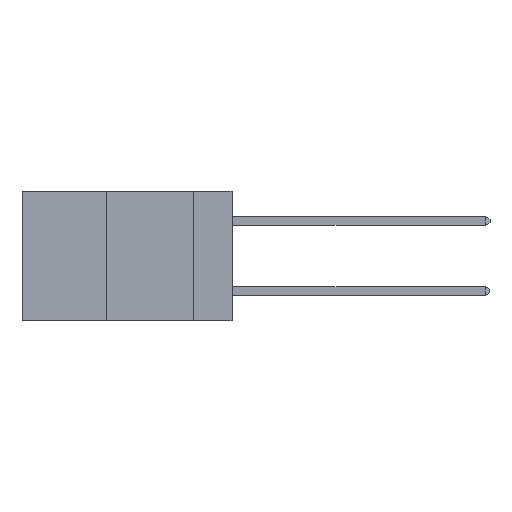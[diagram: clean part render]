
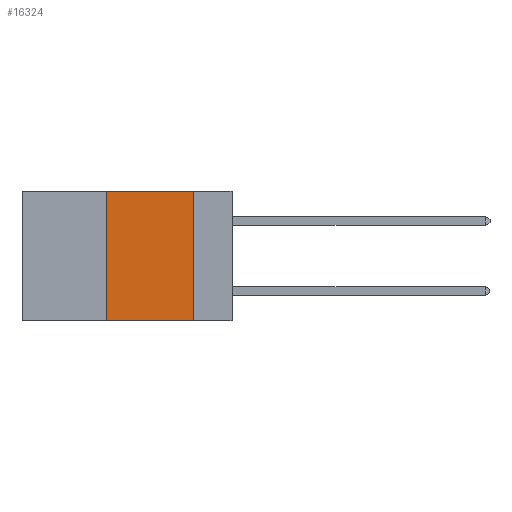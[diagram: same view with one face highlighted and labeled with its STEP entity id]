
A CAD part, left-side view. The second image highlights one B-rep face of the part: STEP entity #16324.
In plain terms, the highlighted planar face has unit normal (-1, 0, 0).
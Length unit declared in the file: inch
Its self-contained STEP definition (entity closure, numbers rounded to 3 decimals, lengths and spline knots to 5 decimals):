
#445 = VECTOR ( 'NONE', #5398, 39.37008 ) ;
#1296 = EDGE_CURVE ( 'NONE', #1911, #14164, #7550, .T. ) ;
#1616 = CARTESIAN_POINT ( 'NONE',  ( 0., 0.6, 0. ) ) ;
#1772 = EDGE_CURVE ( 'NONE', #3666, #14164, #14165, .T. ) ;
#1850 = VERTEX_POINT ( 'NONE', #12374 ) ;
#1911 = VERTEX_POINT ( 'NONE', #6302 ) ;
#2642 = ORIENTED_EDGE ( 'NONE', *, *, #4740, .F. ) ;
#2652 = DIRECTION ( 'NONE',  ( 0., 0., -1. ) ) ;
#3666 = VERTEX_POINT ( 'NONE', #14244 ) ;
#4740 = EDGE_CURVE ( 'NONE', #1850, #3666, #12493, .T. ) ;
#5086 = CARTESIAN_POINT ( 'NONE',  ( 0., 0.11, 0. ) ) ;
#5298 = EDGE_CURVE ( 'NONE', #1911, #1850, #8020, .T. ) ;
#5398 = DIRECTION ( 'NONE',  ( 0., 0., 1. ) ) ;
#5422 = FACE_OUTER_BOUND ( 'NONE', #7669, .T. ) ;
#6302 = CARTESIAN_POINT ( 'NONE',  ( 0., 0.36, -0.37 ) ) ;
#6585 = CARTESIAN_POINT ( 'NONE',  ( 0., 0.6, -0.37 ) ) ;
#7138 = CARTESIAN_POINT ( 'NONE',  ( 0., 0.6, 0. ) ) ;
#7550 = LINE ( 'NONE', #6585, #13780 ) ;
#7669 = EDGE_LOOP ( 'NONE', ( #15383, #2642, #14683, #8000 ) ) ;
#8000 = ORIENTED_EDGE ( 'NONE', *, *, #1296, .T. ) ;
#8020 = LINE ( 'NONE', #11987, #445 ) ;
#8442 = DIRECTION ( 'NONE',  ( 0., 0., -1. ) ) ;
#8859 = VECTOR ( 'NONE', #14699, 39.37008 ) ;
#9919 = DIRECTION ( 'NONE',  ( 0., -1., 0. ) ) ;
#11987 = CARTESIAN_POINT ( 'NONE',  ( 0., 0.36, 0. ) ) ;
#12374 = CARTESIAN_POINT ( 'NONE',  ( 0., 0.36, 0. ) ) ;
#12493 = LINE ( 'NONE', #1616, #8859 ) ;
#13780 = VECTOR ( 'NONE', #9919, 39.37008 ) ;
#13957 = AXIS2_PLACEMENT_3D ( 'NONE', #7138, #15830, #8442 ) ;
#14164 = VERTEX_POINT ( 'NONE', #15225 ) ;
#14165 = LINE ( 'NONE', #5086, #14556 ) ;
#14244 = CARTESIAN_POINT ( 'NONE',  ( 0., 0.11, 0. ) ) ;
#14556 = VECTOR ( 'NONE', #2652, 39.37008 ) ;
#14606 = PLANE ( 'NONE',  #13957 ) ;
#14683 = ORIENTED_EDGE ( 'NONE', *, *, #5298, .F. ) ;
#14699 = DIRECTION ( 'NONE',  ( 0., -1., 0. ) ) ;
#15225 = CARTESIAN_POINT ( 'NONE',  ( 0., 0.11, -0.37 ) ) ;
#15383 = ORIENTED_EDGE ( 'NONE', *, *, #1772, .F. ) ;
#15830 = DIRECTION ( 'NONE',  ( 1., 0., 0. ) ) ;
#16324 = ADVANCED_FACE ( 'NONE', ( #5422 ), #14606, .F. ) ;
